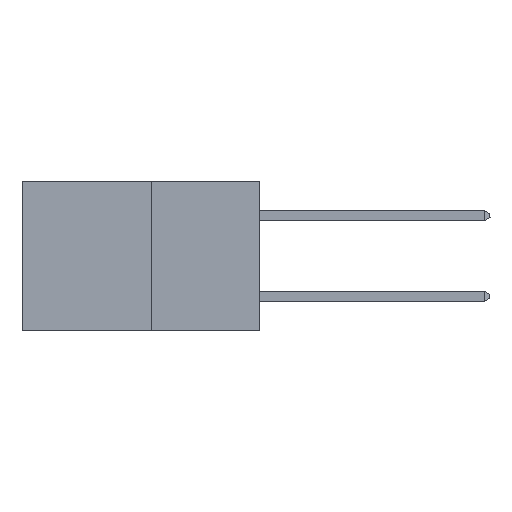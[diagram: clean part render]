
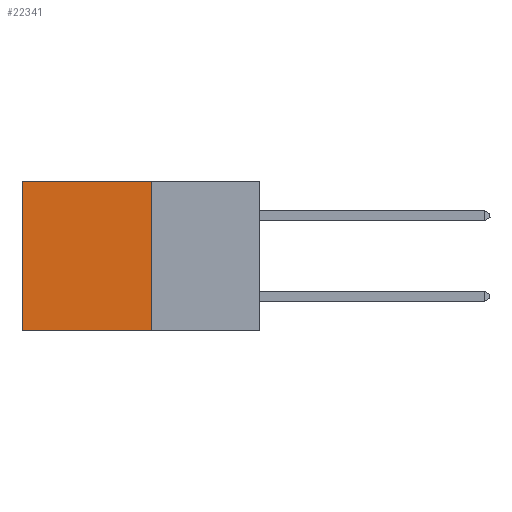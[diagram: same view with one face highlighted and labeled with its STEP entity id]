
A CAD part, left-side view. The second image highlights one B-rep face of the part: STEP entity #22341.
In plain terms, the highlighted planar face has unit normal (-1, 0, 0).
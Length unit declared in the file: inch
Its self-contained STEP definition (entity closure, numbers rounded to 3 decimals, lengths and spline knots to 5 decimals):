
#726 = DIRECTION ( 'NONE',  ( 0., 0., -1. ) ) ;
#803 = ORIENTED_EDGE ( 'NONE', *, *, #17667, .T. ) ;
#1909 = LINE ( 'NONE', #3138, #13141 ) ;
#2901 = LINE ( 'NONE', #23087, #8883 ) ;
#3138 = CARTESIAN_POINT ( 'NONE',  ( 0.277, 0.27, 0. ) ) ;
#3785 = EDGE_CURVE ( 'NONE', #22684, #19485, #9673, .T. ) ;
#4139 = VERTEX_POINT ( 'NONE', #23212 ) ;
#5347 = AXIS2_PLACEMENT_3D ( 'NONE', #20233, #6932, #22445 ) ;
#5348 = DIRECTION ( 'NONE',  ( 0., 1., 0. ) ) ;
#6932 = DIRECTION ( 'NONE',  ( 1., 0., 0. ) ) ;
#7381 = ORIENTED_EDGE ( 'NONE', *, *, #3785, .F. ) ;
#8883 = VECTOR ( 'NONE', #12096, 39.37008 ) ;
#9673 = LINE ( 'NONE', #28185, #14140 ) ;
#11026 = FACE_OUTER_BOUND ( 'NONE', #22099, .T. ) ;
#11037 = EDGE_CURVE ( 'NONE', #14549, #19485, #2901, .T. ) ;
#11930 = CARTESIAN_POINT ( 'NONE',  ( 0.277, 0.27, -0.37 ) ) ;
#11986 = ORIENTED_EDGE ( 'NONE', *, *, #28295, .F. ) ;
#12096 = DIRECTION ( 'NONE',  ( 0., 0., -1. ) ) ;
#13141 = VECTOR ( 'NONE', #5348, 39.37008 ) ;
#13432 = CARTESIAN_POINT ( 'NONE',  ( 0.277, 0.59, -0.37 ) ) ;
#14140 = VECTOR ( 'NONE', #23876, 39.37008 ) ;
#14549 = VERTEX_POINT ( 'NONE', #16949 ) ;
#16861 = CARTESIAN_POINT ( 'NONE',  ( 0.277, 0.27, -0.37 ) ) ;
#16949 = CARTESIAN_POINT ( 'NONE',  ( 0.277, 0.59, 0. ) ) ;
#17667 = EDGE_CURVE ( 'NONE', #4139, #14549, #1909, .T. ) ;
#19485 = VERTEX_POINT ( 'NONE', #13432 ) ;
#19678 = VECTOR ( 'NONE', #726, 39.37008 ) ;
#20233 = CARTESIAN_POINT ( 'NONE',  ( 0.277, 0.27, -0.37 ) ) ;
#20403 = LINE ( 'NONE', #11930, #19678 ) ;
#22099 = EDGE_LOOP ( 'NONE', ( #27855, #7381, #11986, #803 ) ) ;
#22341 = ADVANCED_FACE ( 'NONE', ( #11026 ), #24524, .F. ) ;
#22445 = DIRECTION ( 'NONE',  ( 0., 0., -1. ) ) ;
#22684 = VERTEX_POINT ( 'NONE', #16861 ) ;
#23087 = CARTESIAN_POINT ( 'NONE',  ( 0.277, 0.59, -0.37 ) ) ;
#23212 = CARTESIAN_POINT ( 'NONE',  ( 0.277, 0.27, 0. ) ) ;
#23876 = DIRECTION ( 'NONE',  ( 0., 1., 0. ) ) ;
#24524 = PLANE ( 'NONE',  #5347 ) ;
#27855 = ORIENTED_EDGE ( 'NONE', *, *, #11037, .T. ) ;
#28185 = CARTESIAN_POINT ( 'NONE',  ( 0.277, 0.27, -0.37 ) ) ;
#28295 = EDGE_CURVE ( 'NONE', #4139, #22684, #20403, .T. ) ;
